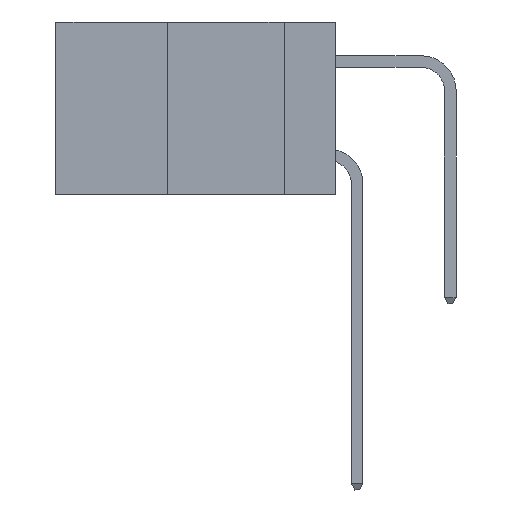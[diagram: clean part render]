
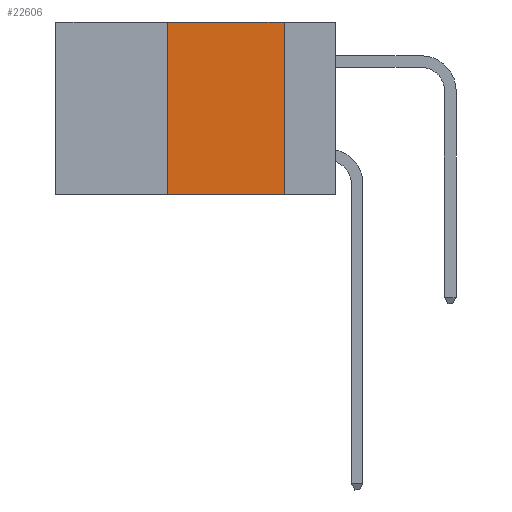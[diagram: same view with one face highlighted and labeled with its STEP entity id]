
A CAD part, left-side view. The second image highlights one B-rep face of the part: STEP entity #22606.
In plain terms, the highlighted planar face has unit normal (-1, 0, 0).
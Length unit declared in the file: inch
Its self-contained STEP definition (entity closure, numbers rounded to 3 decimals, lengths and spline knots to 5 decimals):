
#291 = PLANE ( 'NONE',  #16571 ) ;
#353 = CARTESIAN_POINT ( 'NONE',  ( 0., 0.6, -0.37 ) ) ;
#409 = CARTESIAN_POINT ( 'NONE',  ( 0., 0.36, 0. ) ) ;
#1667 = CARTESIAN_POINT ( 'NONE',  ( 0., 0.36, 0. ) ) ;
#2226 = DIRECTION ( 'NONE',  ( 1., 0., 0. ) ) ;
#2966 = ORIENTED_EDGE ( 'NONE', *, *, #7261, .F. ) ;
#3603 = EDGE_CURVE ( 'NONE', #21215, #10318, #11269, .T. ) ;
#4566 = EDGE_CURVE ( 'NONE', #10318, #16952, #22386, .T. ) ;
#5166 = LINE ( 'NONE', #353, #20628 ) ;
#5786 = DIRECTION ( 'NONE',  ( 0., 0., 1. ) ) ;
#5797 = DIRECTION ( 'NONE',  ( 0., -1., 0. ) ) ;
#5988 = CARTESIAN_POINT ( 'NONE',  ( 0., 0.11, 0. ) ) ;
#7261 = EDGE_CURVE ( 'NONE', #16952, #19221, #8235, .T. ) ;
#7402 = FACE_OUTER_BOUND ( 'NONE', #20626, .T. ) ;
#7639 = DIRECTION ( 'NONE',  ( 0., -1., 0. ) ) ;
#8235 = LINE ( 'NONE', #5988, #13650 ) ;
#8814 = CARTESIAN_POINT ( 'NONE',  ( 0., 0.11, 0. ) ) ;
#10318 = VERTEX_POINT ( 'NONE', #1667 ) ;
#11269 = LINE ( 'NONE', #409, #17309 ) ;
#11446 = DIRECTION ( 'NONE',  ( 0., 0., -1. ) ) ;
#11454 = VECTOR ( 'NONE', #7639, 39.37008 ) ;
#13650 = VECTOR ( 'NONE', #16605, 39.37008 ) ;
#14436 = ORIENTED_EDGE ( 'NONE', *, *, #4566, .F. ) ;
#16571 = AXIS2_PLACEMENT_3D ( 'NONE', #20534, #2226, #11446 ) ;
#16605 = DIRECTION ( 'NONE',  ( 0., 0., -1. ) ) ;
#16952 = VERTEX_POINT ( 'NONE', #8814 ) ;
#17309 = VECTOR ( 'NONE', #5786, 39.37008 ) ;
#18333 = CARTESIAN_POINT ( 'NONE',  ( 0., 0.6, 0. ) ) ;
#18809 = CARTESIAN_POINT ( 'NONE',  ( 0., 0.36, -0.37 ) ) ;
#19221 = VERTEX_POINT ( 'NONE', #19554 ) ;
#19554 = CARTESIAN_POINT ( 'NONE',  ( 0., 0.11, -0.37 ) ) ;
#20534 = CARTESIAN_POINT ( 'NONE',  ( 0., 0.6, 0. ) ) ;
#20626 = EDGE_LOOP ( 'NONE', ( #2966, #14436, #22494, #23467 ) ) ;
#20628 = VECTOR ( 'NONE', #5797, 39.37008 ) ;
#21163 = EDGE_CURVE ( 'NONE', #21215, #19221, #5166, .T. ) ;
#21215 = VERTEX_POINT ( 'NONE', #18809 ) ;
#22386 = LINE ( 'NONE', #18333, #11454 ) ;
#22494 = ORIENTED_EDGE ( 'NONE', *, *, #3603, .F. ) ;
#22606 = ADVANCED_FACE ( 'NONE', ( #7402 ), #291, .F. ) ;
#23467 = ORIENTED_EDGE ( 'NONE', *, *, #21163, .T. ) ;
